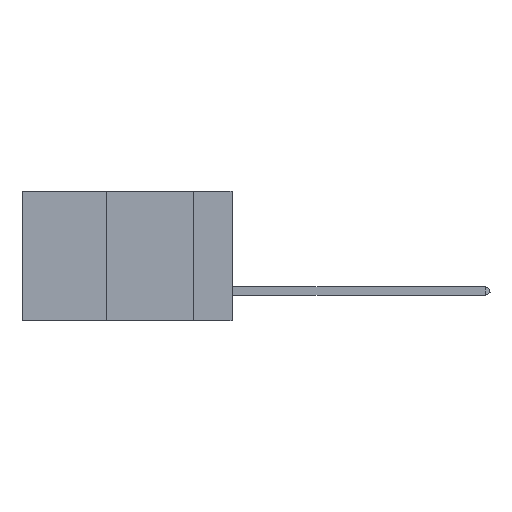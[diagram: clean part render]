
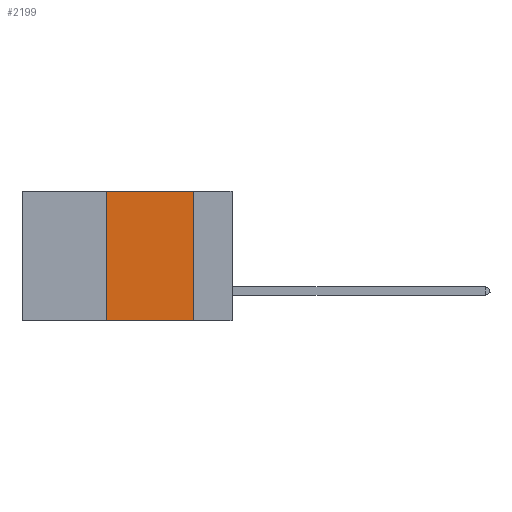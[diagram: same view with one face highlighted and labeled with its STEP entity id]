
A CAD part, left-side view. The second image highlights one B-rep face of the part: STEP entity #2199.
In plain terms, the highlighted planar face has unit normal (-1, 0, 0).
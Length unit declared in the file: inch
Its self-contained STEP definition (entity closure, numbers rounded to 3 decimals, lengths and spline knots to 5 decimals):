
#472 = AXIS2_PLACEMENT_3D ( 'NONE', #24095, #1072, #24230 ) ;
#506 = CARTESIAN_POINT ( 'NONE',  ( 0., 0.11, 0. ) ) ;
#623 = DIRECTION ( 'NONE',  ( 0., 0., -1. ) ) ;
#891 = VECTOR ( 'NONE', #15205, 39.37008 ) ;
#1072 = DIRECTION ( 'NONE',  ( 1., 0., 0. ) ) ;
#2111 = EDGE_CURVE ( 'NONE', #7291, #26217, #15072, .T. ) ;
#2139 = CARTESIAN_POINT ( 'NONE',  ( 0., 0.36, 0. ) ) ;
#2199 = ADVANCED_FACE ( 'NONE', ( #11445 ), #23702, .F. ) ;
#2467 = VERTEX_POINT ( 'NONE', #506 ) ;
#2632 = LINE ( 'NONE', #20976, #2927 ) ;
#2927 = VECTOR ( 'NONE', #623, 39.37008 ) ;
#2981 = CARTESIAN_POINT ( 'NONE',  ( 0., 0.36, -0.37 ) ) ;
#3089 = CARTESIAN_POINT ( 'NONE',  ( 0., 0.6, -0.37 ) ) ;
#4304 = ORIENTED_EDGE ( 'NONE', *, *, #26053, .F. ) ;
#5136 = EDGE_CURVE ( 'NONE', #2467, #26217, #2632, .T. ) ;
#7291 = VERTEX_POINT ( 'NONE', #2981 ) ;
#7333 = DIRECTION ( 'NONE',  ( 0., 0., 1. ) ) ;
#7336 = VECTOR ( 'NONE', #16593, 39.37008 ) ;
#8830 = ORIENTED_EDGE ( 'NONE', *, *, #2111, .T. ) ;
#9791 = EDGE_CURVE ( 'NONE', #23251, #2467, #22681, .T. ) ;
#10156 = VECTOR ( 'NONE', #7333, 39.37008 ) ;
#11189 = EDGE_LOOP ( 'NONE', ( #17848, #22337, #4304, #8830 ) ) ;
#11445 = FACE_OUTER_BOUND ( 'NONE', #11189, .T. ) ;
#12039 = CARTESIAN_POINT ( 'NONE',  ( 0., 0.6, 0. ) ) ;
#15072 = LINE ( 'NONE', #3089, #891 ) ;
#15205 = DIRECTION ( 'NONE',  ( 0., -1., 0. ) ) ;
#16593 = DIRECTION ( 'NONE',  ( 0., -1., 0. ) ) ;
#17848 = ORIENTED_EDGE ( 'NONE', *, *, #5136, .F. ) ;
#19598 = CARTESIAN_POINT ( 'NONE',  ( 0., 0.36, 0. ) ) ;
#20267 = CARTESIAN_POINT ( 'NONE',  ( 0., 0.11, -0.37 ) ) ;
#20976 = CARTESIAN_POINT ( 'NONE',  ( 0., 0.11, 0. ) ) ;
#22337 = ORIENTED_EDGE ( 'NONE', *, *, #9791, .F. ) ;
#22681 = LINE ( 'NONE', #12039, #7336 ) ;
#23251 = VERTEX_POINT ( 'NONE', #2139 ) ;
#23652 = LINE ( 'NONE', #19598, #10156 ) ;
#23702 = PLANE ( 'NONE',  #472 ) ;
#24095 = CARTESIAN_POINT ( 'NONE',  ( 0., 0.6, 0. ) ) ;
#24230 = DIRECTION ( 'NONE',  ( 0., 0., -1. ) ) ;
#26053 = EDGE_CURVE ( 'NONE', #7291, #23251, #23652, .T. ) ;
#26217 = VERTEX_POINT ( 'NONE', #20267 ) ;
